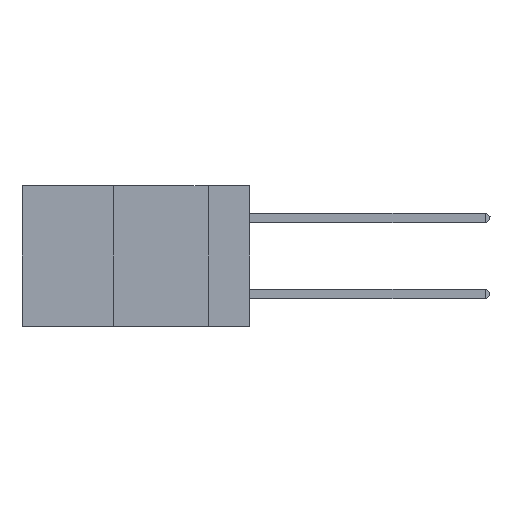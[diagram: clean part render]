
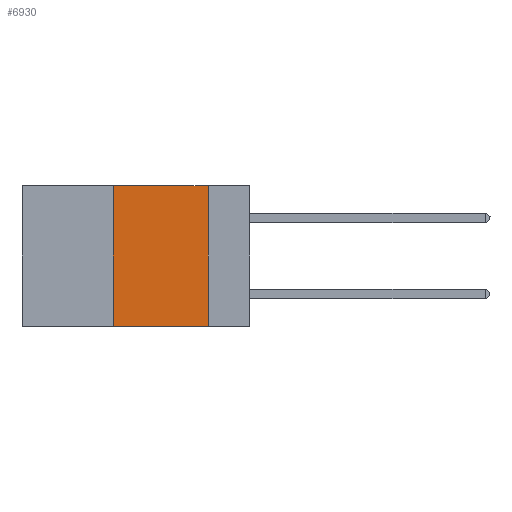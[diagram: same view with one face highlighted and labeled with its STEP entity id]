
A CAD part, left-side view. The second image highlights one B-rep face of the part: STEP entity #6930.
In plain terms, the highlighted planar face has unit normal (-1, 0, 0).
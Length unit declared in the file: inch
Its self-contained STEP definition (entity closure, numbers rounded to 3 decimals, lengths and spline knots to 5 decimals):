
#130 = CARTESIAN_POINT ( 'NONE',  ( 0., 0.6, 0. ) ) ;
#1215 = PLANE ( 'NONE',  #4881 ) ;
#2835 = LINE ( 'NONE', #130, #6487 ) ;
#3048 = EDGE_CURVE ( 'NONE', #12126, #8976, #15175, .T. ) ;
#3402 = ORIENTED_EDGE ( 'NONE', *, *, #22060, .F. ) ;
#3946 = VECTOR ( 'NONE', #5351, 39.37008 ) ;
#4752 = LINE ( 'NONE', #17502, #13310 ) ;
#4881 = AXIS2_PLACEMENT_3D ( 'NONE', #7170, #22001, #24131 ) ;
#5351 = DIRECTION ( 'NONE',  ( 0., 0., -1. ) ) ;
#6477 = DIRECTION ( 'NONE',  ( 0., -1., 0. ) ) ;
#6487 = VECTOR ( 'NONE', #6808, 39.37008 ) ;
#6706 = EDGE_CURVE ( 'NONE', #19518, #12126, #2835, .T. ) ;
#6808 = DIRECTION ( 'NONE',  ( 0., -1., 0. ) ) ;
#6930 = ADVANCED_FACE ( 'NONE', ( #10074 ), #1215, .F. ) ;
#7170 = CARTESIAN_POINT ( 'NONE',  ( 0., 0.6, 0. ) ) ;
#7234 = CARTESIAN_POINT ( 'NONE',  ( 0., 0.11, -0.37 ) ) ;
#7596 = ORIENTED_EDGE ( 'NONE', *, *, #9367, .T. ) ;
#8976 = VERTEX_POINT ( 'NONE', #7234 ) ;
#9367 = EDGE_CURVE ( 'NONE', #26287, #8976, #16585, .T. ) ;
#9765 = CARTESIAN_POINT ( 'NONE',  ( 0., 0.36, -0.37 ) ) ;
#10074 = FACE_OUTER_BOUND ( 'NONE', #13253, .T. ) ;
#11505 = ORIENTED_EDGE ( 'NONE', *, *, #3048, .F. ) ;
#12061 = ORIENTED_EDGE ( 'NONE', *, *, #6706, .F. ) ;
#12126 = VERTEX_POINT ( 'NONE', #12649 ) ;
#12649 = CARTESIAN_POINT ( 'NONE',  ( 0., 0.11, 0. ) ) ;
#13253 = EDGE_LOOP ( 'NONE', ( #11505, #12061, #3402, #7596 ) ) ;
#13310 = VECTOR ( 'NONE', #21983, 39.37008 ) ;
#15175 = LINE ( 'NONE', #24347, #3946 ) ;
#16585 = LINE ( 'NONE', #19230, #19252 ) ;
#17502 = CARTESIAN_POINT ( 'NONE',  ( 0., 0.36, 0. ) ) ;
#19230 = CARTESIAN_POINT ( 'NONE',  ( 0., 0.6, -0.37 ) ) ;
#19252 = VECTOR ( 'NONE', #6477, 39.37008 ) ;
#19518 = VERTEX_POINT ( 'NONE', #20161 ) ;
#20161 = CARTESIAN_POINT ( 'NONE',  ( 0., 0.36, 0. ) ) ;
#21983 = DIRECTION ( 'NONE',  ( 0., 0., 1. ) ) ;
#22001 = DIRECTION ( 'NONE',  ( 1., 0., 0. ) ) ;
#22060 = EDGE_CURVE ( 'NONE', #26287, #19518, #4752, .T. ) ;
#24131 = DIRECTION ( 'NONE',  ( 0., 0., -1. ) ) ;
#24347 = CARTESIAN_POINT ( 'NONE',  ( 0., 0.11, 0. ) ) ;
#26287 = VERTEX_POINT ( 'NONE', #9765 ) ;
